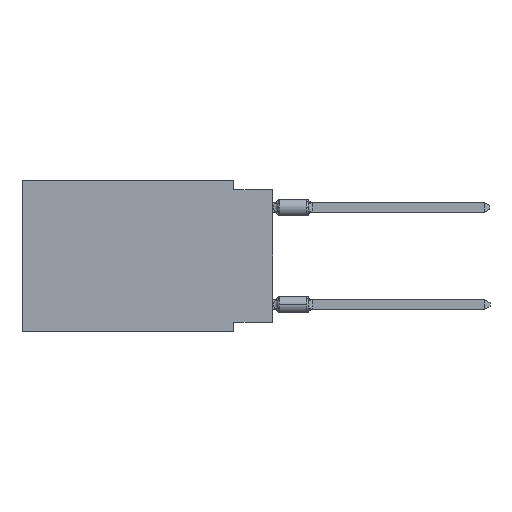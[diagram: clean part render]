
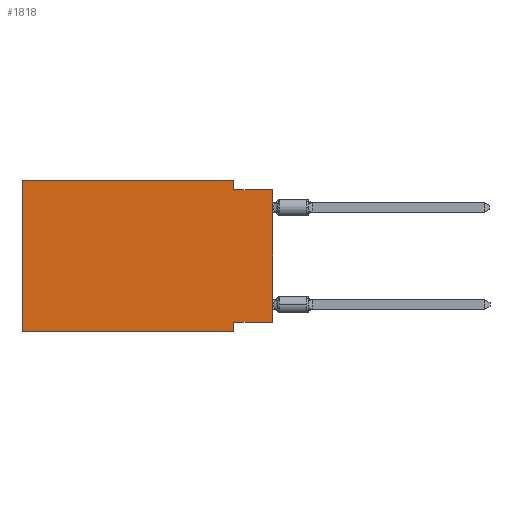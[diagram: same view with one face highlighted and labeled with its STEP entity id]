
A CAD part, left-side view. The second image highlights one B-rep face of the part: STEP entity #1818.
In plain terms, the highlighted planar face has unit normal (-1, 0, 0).
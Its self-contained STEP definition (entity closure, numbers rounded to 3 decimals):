
#24 = LINE ( 'NONE', #3368, #20690 ) ;
#1171 = LINE ( 'NONE', #4555, #3196 ) ;
#1489 = AXIS2_PLACEMENT_3D ( 'NONE', #7537, #5731, #12708 ) ;
#1597 = EDGE_CURVE ( 'NONE', #6531, #20984, #18136, .T. ) ;
#1636 = VERTEX_POINT ( 'NONE', #18241 ) ;
#1649 = VERTEX_POINT ( 'NONE', #16509 ) ;
#1818 = ADVANCED_FACE ( 'NONE', ( #12608 ), #4304, .F. ) ;
#1913 = VERTEX_POINT ( 'NONE', #3186 ) ;
#2196 = EDGE_CURVE ( 'NONE', #10885, #20984, #3619, .T. ) ;
#2205 = DIRECTION ( 'NONE',  ( 0., 0., -1. ) ) ;
#2841 = VERTEX_POINT ( 'NONE', #14386 ) ;
#3019 = DIRECTION ( 'NONE',  ( 0., 1., 0. ) ) ;
#3089 = LINE ( 'NONE', #16293, #5592 ) ;
#3186 = CARTESIAN_POINT ( 'NONE',  ( 0., 16.383, 0. ) ) ;
#3196 = VECTOR ( 'NONE', #3019, 1000. ) ;
#3326 = DIRECTION ( 'NONE',  ( 0., -1., 0. ) ) ;
#3368 = CARTESIAN_POINT ( 'NONE',  ( 0., 2.54, 0. ) ) ;
#3424 = CARTESIAN_POINT ( 'NONE',  ( 0., 2.54, -9.906 ) ) ;
#3558 = EDGE_CURVE ( 'NONE', #1913, #1649, #3089, .T. ) ;
#3619 = LINE ( 'NONE', #3723, #20142 ) ;
#3723 = CARTESIAN_POINT ( 'NONE',  ( 0., 2.54, -9.906 ) ) ;
#3949 = ORIENTED_EDGE ( 'NONE', *, *, #20549, .T. ) ;
#4016 = DIRECTION ( 'NONE',  ( 0., 0., 1. ) ) ;
#4163 = ORIENTED_EDGE ( 'NONE', *, *, #11757, .F. ) ;
#4304 = PLANE ( 'NONE',  #1489 ) ;
#4555 = CARTESIAN_POINT ( 'NONE',  ( 0., 0., -9.271 ) ) ;
#5031 = ORIENTED_EDGE ( 'NONE', *, *, #3558, .F. ) ;
#5592 = VECTOR ( 'NONE', #8291, 1000. ) ;
#5652 = LINE ( 'NONE', #20626, #17818 ) ;
#5731 = DIRECTION ( 'NONE',  ( 1., 0., 0. ) ) ;
#5864 = VECTOR ( 'NONE', #17169, 1000. ) ;
#6013 = VECTOR ( 'NONE', #3326, 1000. ) ;
#6052 = EDGE_LOOP ( 'NONE', ( #3949, #8299, #15241, #5031, #4163, #9504, #16994, #19519 ) ) ;
#6362 = CARTESIAN_POINT ( 'NONE',  ( 0., 0., -0.635 ) ) ;
#6531 = VERTEX_POINT ( 'NONE', #13367 ) ;
#6717 = CARTESIAN_POINT ( 'NONE',  ( 0., 0., 0. ) ) ;
#7519 = EDGE_CURVE ( 'NONE', #2841, #10597, #18782, .T. ) ;
#7537 = CARTESIAN_POINT ( 'NONE',  ( 0., 16.383, 0. ) ) ;
#8291 = DIRECTION ( 'NONE',  ( 0., -1., 0. ) ) ;
#8299 = ORIENTED_EDGE ( 'NONE', *, *, #7519, .F. ) ;
#9457 = CARTESIAN_POINT ( 'NONE',  ( 0., 2.54, -9.271 ) ) ;
#9504 = ORIENTED_EDGE ( 'NONE', *, *, #1597, .T. ) ;
#10597 = VERTEX_POINT ( 'NONE', #6362 ) ;
#10885 = VERTEX_POINT ( 'NONE', #9457 ) ;
#11757 = EDGE_CURVE ( 'NONE', #6531, #1913, #5652, .T. ) ;
#12608 = FACE_OUTER_BOUND ( 'NONE', #6052, .T. ) ;
#12708 = DIRECTION ( 'NONE',  ( 0., 0., -1. ) ) ;
#13211 = DIRECTION ( 'NONE',  ( 0., 0., -1. ) ) ;
#13367 = CARTESIAN_POINT ( 'NONE',  ( 0., 16.383, -9.906 ) ) ;
#14287 = VECTOR ( 'NONE', #19876, 1000. ) ;
#14386 = CARTESIAN_POINT ( 'NONE',  ( 0., 2.54, -0.635 ) ) ;
#15241 = ORIENTED_EDGE ( 'NONE', *, *, #18530, .F. ) ;
#16293 = CARTESIAN_POINT ( 'NONE',  ( 0., 16.383, 0. ) ) ;
#16509 = CARTESIAN_POINT ( 'NONE',  ( 0., 2.54, 0. ) ) ;
#16641 = LINE ( 'NONE', #6717, #14287 ) ;
#16994 = ORIENTED_EDGE ( 'NONE', *, *, #2196, .F. ) ;
#17169 = DIRECTION ( 'NONE',  ( 0., -1., 0. ) ) ;
#17818 = VECTOR ( 'NONE', #4016, 1000. ) ;
#18136 = LINE ( 'NONE', #19420, #6013 ) ;
#18241 = CARTESIAN_POINT ( 'NONE',  ( 0., 0., -9.271 ) ) ;
#18530 = EDGE_CURVE ( 'NONE', #1649, #2841, #24, .T. ) ;
#18782 = LINE ( 'NONE', #20390, #5864 ) ;
#19233 = EDGE_CURVE ( 'NONE', #1636, #10885, #1171, .T. ) ;
#19420 = CARTESIAN_POINT ( 'NONE',  ( 0., 16.383, -9.906 ) ) ;
#19519 = ORIENTED_EDGE ( 'NONE', *, *, #19233, .F. ) ;
#19876 = DIRECTION ( 'NONE',  ( 0., 0., 1. ) ) ;
#20142 = VECTOR ( 'NONE', #2205, 1000. ) ;
#20390 = CARTESIAN_POINT ( 'NONE',  ( 0., 0., -0.635 ) ) ;
#20549 = EDGE_CURVE ( 'NONE', #1636, #10597, #16641, .T. ) ;
#20626 = CARTESIAN_POINT ( 'NONE',  ( 0., 16.383, 0. ) ) ;
#20690 = VECTOR ( 'NONE', #13211, 1000. ) ;
#20984 = VERTEX_POINT ( 'NONE', #3424 ) ;
